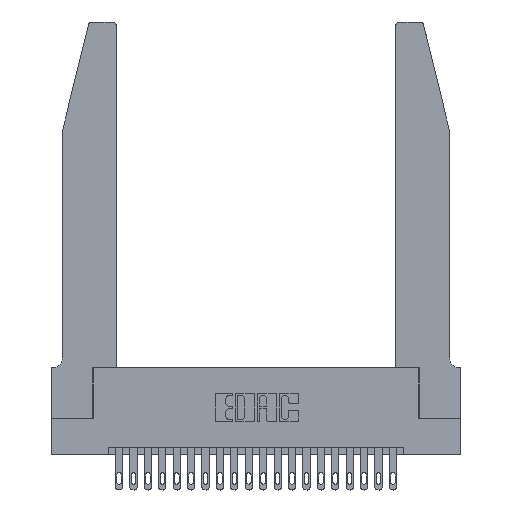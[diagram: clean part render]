
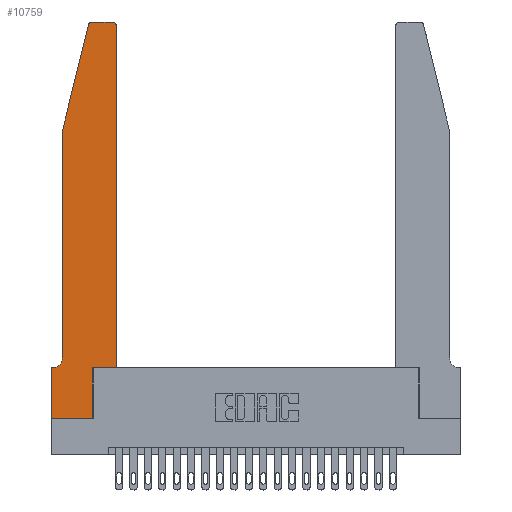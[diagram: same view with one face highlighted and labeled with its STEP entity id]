
A CAD part, top view. The second image highlights one B-rep face of the part: STEP entity #10759.
In plain terms, the highlighted planar face has unit normal (0, 0, 1).
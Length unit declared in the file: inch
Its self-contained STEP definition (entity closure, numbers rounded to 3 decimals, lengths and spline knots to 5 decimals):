
#41 = DIRECTION ( 'NONE',  ( 1., 0., 0. ) ) ;
#316 = LINE ( 'NONE', #4039, #3082 ) ;
#548 = CARTESIAN_POINT ( 'NONE',  ( 0.0055, 0.42, 0.37 ) ) ;
#885 = CIRCLE ( 'NONE', #17965, 0.03 ) ;
#915 = CARTESIAN_POINT ( 'NONE',  ( 0., 0.35, 0.37 ) ) ;
#1844 = CIRCLE ( 'NONE', #18840, 0.07 ) ;
#2167 = CARTESIAN_POINT ( 'NONE',  ( 0.0755, 0.35, 0.37 ) ) ;
#3006 = VECTOR ( 'NONE', #14854, 39.37008 ) ;
#3082 = VECTOR ( 'NONE', #9624, 39.37008 ) ;
#3424 = LINE ( 'NONE', #14727, #16142 ) ;
#3740 = CARTESIAN_POINT ( 'NONE',  ( 0.4505, 0.35, 0.37 ) ) ;
#3785 = DIRECTION ( 'NONE',  ( 0., 0., 1. ) ) ;
#3884 = DIRECTION ( 'NONE',  ( 0., -1., 0. ) ) ;
#4039 = CARTESIAN_POINT ( 'NONE',  ( 0.2865, 0.35, 0.37 ) ) ;
#4077 = CARTESIAN_POINT ( 'NONE',  ( 0.2865, 0.35, 0.37 ) ) ;
#4310 = DIRECTION ( 'NONE',  ( 0., 0., -1. ) ) ;
#4453 = CIRCLE ( 'NONE', #13825, 0.03 ) ;
#4655 = DIRECTION ( 'NONE',  ( 0., 0., 1. ) ) ;
#4730 = DIRECTION ( 'NONE',  ( 1., 0., 0. ) ) ;
#4978 = DIRECTION ( 'NONE',  ( 1., 0., 0. ) ) ;
#5341 = EDGE_CURVE ( 'NONE', #12155, #19027, #4453, .T. ) ;
#5606 = VECTOR ( 'NONE', #8589, 39.37008 ) ;
#5764 = LINE ( 'NONE', #6714, #8574 ) ;
#6089 = VERTEX_POINT ( 'NONE', #3740 ) ;
#6311 = CARTESIAN_POINT ( 'NONE',  ( 0.0055, 0.35, 0.37 ) ) ;
#6558 = VERTEX_POINT ( 'NONE', #13499 ) ;
#6675 = LINE ( 'NONE', #23225, #12619 ) ;
#6704 = LINE ( 'NONE', #2167, #21419 ) ;
#6714 = CARTESIAN_POINT ( 'NONE',  ( 0.4505, 0.35, 0.37 ) ) ;
#6730 = CARTESIAN_POINT ( 'NONE',  ( 0., 0., 0.37 ) ) ;
#7065 = EDGE_CURVE ( 'NONE', #10640, #16926, #11570, .T. ) ;
#7832 = CARTESIAN_POINT ( 'NONE',  ( 0.0755, 2., 0.37 ) ) ;
#8250 = ORIENTED_EDGE ( 'NONE', *, *, #10816, .T. ) ;
#8556 = VERTEX_POINT ( 'NONE', #6311 ) ;
#8574 = VECTOR ( 'NONE', #15945, 39.37008 ) ;
#8589 = DIRECTION ( 'NONE',  ( -0.239, -0.971, 0. ) ) ;
#8647 = ORIENTED_EDGE ( 'NONE', *, *, #18745, .T. ) ;
#8904 = DIRECTION ( 'NONE',  ( 1., 0., 0. ) ) ;
#9219 = ORIENTED_EDGE ( 'NONE', *, *, #5341, .T. ) ;
#9406 = DIRECTION ( 'NONE',  ( 0., -1., 0. ) ) ;
#9598 = CARTESIAN_POINT ( 'NONE',  ( 0.0755, 0.42, 0.37 ) ) ;
#9624 = DIRECTION ( 'NONE',  ( 0., 1., 0. ) ) ;
#9878 = EDGE_CURVE ( 'NONE', #16926, #8556, #1844, .T. ) ;
#9986 = EDGE_CURVE ( 'NONE', #19715, #19546, #316, .T. ) ;
#9992 = ORIENTED_EDGE ( 'NONE', *, *, #7065, .T. ) ;
#10206 = ORIENTED_EDGE ( 'NONE', *, *, #12328, .T. ) ;
#10640 = VERTEX_POINT ( 'NONE', #20610 ) ;
#10759 = ADVANCED_FACE ( 'NONE', ( #22031 ), #20684, .T. ) ;
#10813 = LINE ( 'NONE', #19346, #17643 ) ;
#10816 = EDGE_CURVE ( 'NONE', #6558, #20951, #885, .T. ) ;
#10976 = AXIS2_PLACEMENT_3D ( 'NONE', #915, #4655, #4730 ) ;
#11221 = DIRECTION ( 'NONE',  ( -1., 0., 0. ) ) ;
#11483 = DIRECTION ( 'NONE',  ( -1., 0., 0. ) ) ;
#11526 = CARTESIAN_POINT ( 'NONE',  ( 0., 0.35, 0.37 ) ) ;
#11570 = LINE ( 'NONE', #7832, #20049 ) ;
#11781 = CARTESIAN_POINT ( 'NONE',  ( 0.25487, 2.72718, 0.37 ) ) ;
#11812 = ORIENTED_EDGE ( 'NONE', *, *, #18755, .T. ) ;
#12043 = EDGE_CURVE ( 'NONE', #8556, #23278, #6704, .T. ) ;
#12155 = VERTEX_POINT ( 'NONE', #16985 ) ;
#12169 = ORIENTED_EDGE ( 'NONE', *, *, #9986, .T. ) ;
#12328 = EDGE_CURVE ( 'NONE', #20951, #10640, #21397, .T. ) ;
#12619 = VECTOR ( 'NONE', #21506, 39.37008 ) ;
#12850 = CARTESIAN_POINT ( 'NONE',  ( 0.4205, 2.72, 0.37 ) ) ;
#13499 = CARTESIAN_POINT ( 'NONE',  ( 0.284, 2.75, 0.37 ) ) ;
#13545 = EDGE_LOOP ( 'NONE', ( #22631, #8250, #10206, #9992, #18860, #22339, #17953, #20722, #12169, #11812, #8647, #9219 ) ) ;
#13670 = CARTESIAN_POINT ( 'NONE',  ( 0.4205, 2.75, 0.37 ) ) ;
#13809 = EDGE_CURVE ( 'NONE', #20196, #19715, #17136, .T. ) ;
#13825 = AXIS2_PLACEMENT_3D ( 'NONE', #12850, #3785, #41 ) ;
#14230 = DIRECTION ( 'NONE',  ( 0., 0., 1. ) ) ;
#14727 = CARTESIAN_POINT ( 'NONE',  ( 0., 0., 0.37 ) ) ;
#14854 = DIRECTION ( 'NONE',  ( 1., 0., 0. ) ) ;
#15302 = CARTESIAN_POINT ( 'NONE',  ( 0.2865, 0., 0.37 ) ) ;
#15945 = DIRECTION ( 'NONE',  ( 0., 1., 0. ) ) ;
#16142 = VECTOR ( 'NONE', #3884, 39.37008 ) ;
#16741 = EDGE_CURVE ( 'NONE', #23278, #20196, #3424, .T. ) ;
#16926 = VERTEX_POINT ( 'NONE', #9598 ) ;
#16985 = CARTESIAN_POINT ( 'NONE',  ( 0.4505, 2.72, 0.37 ) ) ;
#17136 = LINE ( 'NONE', #6730, #3006 ) ;
#17643 = VECTOR ( 'NONE', #4978, 39.37008 ) ;
#17953 = ORIENTED_EDGE ( 'NONE', *, *, #16741, .T. ) ;
#17965 = AXIS2_PLACEMENT_3D ( 'NONE', #19730, #14230, #8904 ) ;
#18745 = EDGE_CURVE ( 'NONE', #6089, #12155, #5764, .T. ) ;
#18755 = EDGE_CURVE ( 'NONE', #19546, #6089, #10813, .T. ) ;
#18840 = AXIS2_PLACEMENT_3D ( 'NONE', #548, #4310, #11483 ) ;
#18860 = ORIENTED_EDGE ( 'NONE', *, *, #9878, .T. ) ;
#19027 = VERTEX_POINT ( 'NONE', #13670 ) ;
#19346 = CARTESIAN_POINT ( 'NONE',  ( 0.4505, 0.35, 0.37 ) ) ;
#19410 = CARTESIAN_POINT ( 'NONE',  ( 0.0755, 2., 0.37 ) ) ;
#19546 = VERTEX_POINT ( 'NONE', #4077 ) ;
#19715 = VERTEX_POINT ( 'NONE', #15302 ) ;
#19730 = CARTESIAN_POINT ( 'NONE',  ( 0.284, 2.72, 0.37 ) ) ;
#20049 = VECTOR ( 'NONE', #9406, 39.37008 ) ;
#20196 = VERTEX_POINT ( 'NONE', #20777 ) ;
#20610 = CARTESIAN_POINT ( 'NONE',  ( 0.0755, 2., 0.37 ) ) ;
#20684 = PLANE ( 'NONE',  #10976 ) ;
#20722 = ORIENTED_EDGE ( 'NONE', *, *, #13809, .T. ) ;
#20777 = CARTESIAN_POINT ( 'NONE',  ( 0., 0., 0.37 ) ) ;
#20951 = VERTEX_POINT ( 'NONE', #11781 ) ;
#21397 = LINE ( 'NONE', #19410, #5606 ) ;
#21419 = VECTOR ( 'NONE', #11221, 39.37008 ) ;
#21506 = DIRECTION ( 'NONE',  ( -1., 0., 0. ) ) ;
#22031 = FACE_OUTER_BOUND ( 'NONE', #13545, .T. ) ;
#22339 = ORIENTED_EDGE ( 'NONE', *, *, #12043, .T. ) ;
#22631 = ORIENTED_EDGE ( 'NONE', *, *, #22931, .T. ) ;
#22931 = EDGE_CURVE ( 'NONE', #19027, #6558, #6675, .T. ) ;
#23225 = CARTESIAN_POINT ( 'NONE',  ( 0.2605, 2.75, 0.37 ) ) ;
#23278 = VERTEX_POINT ( 'NONE', #11526 ) ;
